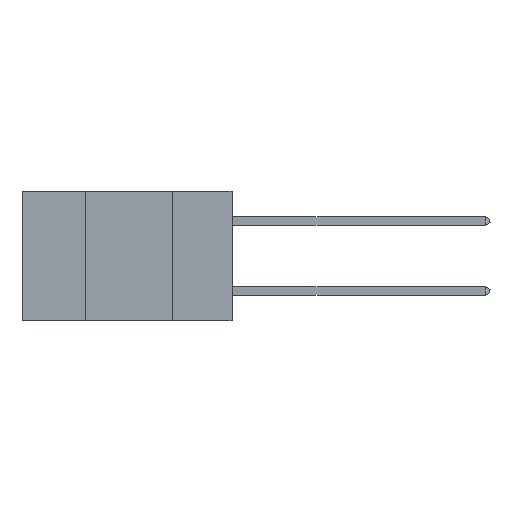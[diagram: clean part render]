
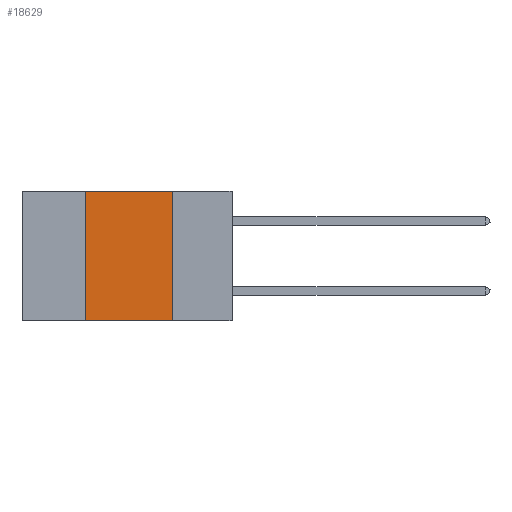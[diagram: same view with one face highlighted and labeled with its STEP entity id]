
A CAD part, left-side view. The second image highlights one B-rep face of the part: STEP entity #18629.
In plain terms, the highlighted planar face has unit normal (-1, 0, 0).
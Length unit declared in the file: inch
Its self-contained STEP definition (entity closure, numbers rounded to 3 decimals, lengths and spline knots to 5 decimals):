
#1490 = VECTOR ( 'NONE', #6979, 39.37008 ) ;
#1900 = VERTEX_POINT ( 'NONE', #8256 ) ;
#2952 = EDGE_CURVE ( 'NONE', #5177, #1900, #9482, .T. ) ;
#2999 = VERTEX_POINT ( 'NONE', #12577 ) ;
#3117 = CARTESIAN_POINT ( 'NONE',  ( 0., 0.6, 0. ) ) ;
#3199 = ORIENTED_EDGE ( 'NONE', *, *, #2952, .F. ) ;
#4725 = DIRECTION ( 'NONE',  ( 0., 0., -1. ) ) ;
#4936 = ORIENTED_EDGE ( 'NONE', *, *, #16488, .F. ) ;
#5177 = VERTEX_POINT ( 'NONE', #6953 ) ;
#5358 = CARTESIAN_POINT ( 'NONE',  ( 0., 0.17, 0. ) ) ;
#6279 = PLANE ( 'NONE',  #14264 ) ;
#6953 = CARTESIAN_POINT ( 'NONE',  ( 0., 0.42, -0.37 ) ) ;
#6979 = DIRECTION ( 'NONE',  ( 0., 0., -1. ) ) ;
#7157 = ORIENTED_EDGE ( 'NONE', *, *, #17801, .T. ) ;
#7579 = CARTESIAN_POINT ( 'NONE',  ( 0., 0.6, 0. ) ) ;
#7737 = CARTESIAN_POINT ( 'NONE',  ( 0., 0.42, 0. ) ) ;
#8256 = CARTESIAN_POINT ( 'NONE',  ( 0., 0.42, 0. ) ) ;
#8479 = VECTOR ( 'NONE', #20303, 39.37008 ) ;
#8641 = VECTOR ( 'NONE', #18515, 39.37008 ) ;
#8818 = CARTESIAN_POINT ( 'NONE',  ( 0., 0.6, -0.37 ) ) ;
#9076 = LINE ( 'NONE', #8818, #20607 ) ;
#9482 = LINE ( 'NONE', #7737, #8479 ) ;
#10092 = LINE ( 'NONE', #5358, #1490 ) ;
#11535 = CARTESIAN_POINT ( 'NONE',  ( 0., 0.17, -0.37 ) ) ;
#12577 = CARTESIAN_POINT ( 'NONE',  ( 0., 0.17, 0. ) ) ;
#14252 = DIRECTION ( 'NONE',  ( 1., 0., 0. ) ) ;
#14264 = AXIS2_PLACEMENT_3D ( 'NONE', #3117, #14252, #4725 ) ;
#16149 = VERTEX_POINT ( 'NONE', #11535 ) ;
#16488 = EDGE_CURVE ( 'NONE', #1900, #2999, #17018, .T. ) ;
#17018 = LINE ( 'NONE', #7579, #8641 ) ;
#17801 = EDGE_CURVE ( 'NONE', #5177, #16149, #9076, .T. ) ;
#18227 = DIRECTION ( 'NONE',  ( 0., -1., 0. ) ) ;
#18362 = EDGE_LOOP ( 'NONE', ( #20239, #4936, #3199, #7157 ) ) ;
#18515 = DIRECTION ( 'NONE',  ( 0., -1., 0. ) ) ;
#18629 = ADVANCED_FACE ( 'NONE', ( #20077 ), #6279, .F. ) ;
#20077 = FACE_OUTER_BOUND ( 'NONE', #18362, .T. ) ;
#20239 = ORIENTED_EDGE ( 'NONE', *, *, #20288, .F. ) ;
#20288 = EDGE_CURVE ( 'NONE', #2999, #16149, #10092, .T. ) ;
#20303 = DIRECTION ( 'NONE',  ( 0., 0., 1. ) ) ;
#20607 = VECTOR ( 'NONE', #18227, 39.37008 ) ;
